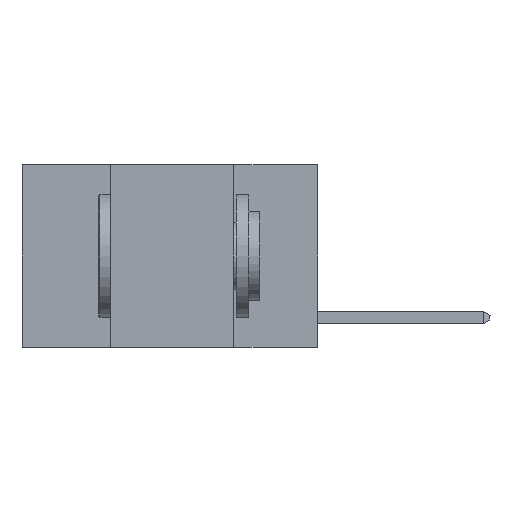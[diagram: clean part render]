
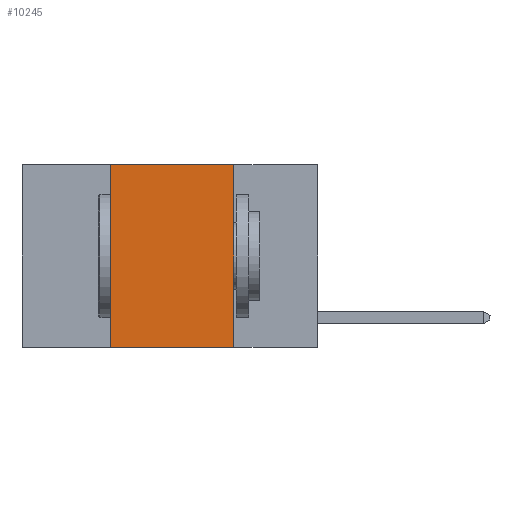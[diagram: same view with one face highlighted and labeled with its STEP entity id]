
A CAD part, left-side view. The second image highlights one B-rep face of the part: STEP entity #10245.
In plain terms, the highlighted planar face has unit normal (-1, 0, 0).
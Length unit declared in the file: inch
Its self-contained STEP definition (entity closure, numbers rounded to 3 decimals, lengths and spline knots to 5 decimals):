
#399 = CARTESIAN_POINT ( 'NONE',  ( 0., 0.42, 0. ) ) ;
#499 = VECTOR ( 'NONE', #5237, 39.37008 ) ;
#953 = ORIENTED_EDGE ( 'NONE', *, *, #14781, .F. ) ;
#2214 = EDGE_CURVE ( 'NONE', #9195, #16380, #9853, .T. ) ;
#2644 = EDGE_CURVE ( 'NONE', #16380, #14195, #6118, .T. ) ;
#5237 = DIRECTION ( 'NONE',  ( 0., 0., 1. ) ) ;
#5583 = VECTOR ( 'NONE', #18920, 39.37008 ) ;
#5860 = DIRECTION ( 'NONE',  ( 0., 0., -1. ) ) ;
#6118 = LINE ( 'NONE', #16441, #20016 ) ;
#6196 = DIRECTION ( 'NONE',  ( 0., -1., 0. ) ) ;
#6877 = CARTESIAN_POINT ( 'NONE',  ( 0., 0.42, -0.37 ) ) ;
#8248 = VERTEX_POINT ( 'NONE', #22944 ) ;
#8418 = LINE ( 'NONE', #15172, #11577 ) ;
#9195 = VERTEX_POINT ( 'NONE', #6877 ) ;
#9631 = ORIENTED_EDGE ( 'NONE', *, *, #11761, .T. ) ;
#9853 = LINE ( 'NONE', #22714, #499 ) ;
#10245 = ADVANCED_FACE ( 'NONE', ( #18081 ), #11135, .F. ) ;
#11135 = PLANE ( 'NONE',  #13983 ) ;
#11577 = VECTOR ( 'NONE', #6196, 39.37008 ) ;
#11761 = EDGE_CURVE ( 'NONE', #9195, #8248, #8418, .T. ) ;
#13805 = ORIENTED_EDGE ( 'NONE', *, *, #2644, .F. ) ;
#13983 = AXIS2_PLACEMENT_3D ( 'NONE', #16657, #20519, #5860 ) ;
#14137 = EDGE_LOOP ( 'NONE', ( #953, #13805, #22212, #9631 ) ) ;
#14195 = VERTEX_POINT ( 'NONE', #18393 ) ;
#14781 = EDGE_CURVE ( 'NONE', #14195, #8248, #20051, .T. ) ;
#15172 = CARTESIAN_POINT ( 'NONE',  ( 0., 0.6, -0.37 ) ) ;
#16380 = VERTEX_POINT ( 'NONE', #399 ) ;
#16441 = CARTESIAN_POINT ( 'NONE',  ( 0., 0.6, 0. ) ) ;
#16657 = CARTESIAN_POINT ( 'NONE',  ( 0., 0.6, 0. ) ) ;
#17093 = CARTESIAN_POINT ( 'NONE',  ( 0., 0.17, 0. ) ) ;
#18081 = FACE_OUTER_BOUND ( 'NONE', #14137, .T. ) ;
#18331 = DIRECTION ( 'NONE',  ( 0., -1., 0. ) ) ;
#18393 = CARTESIAN_POINT ( 'NONE',  ( 0., 0.17, 0. ) ) ;
#18920 = DIRECTION ( 'NONE',  ( 0., 0., -1. ) ) ;
#20016 = VECTOR ( 'NONE', #18331, 39.37008 ) ;
#20051 = LINE ( 'NONE', #17093, #5583 ) ;
#20519 = DIRECTION ( 'NONE',  ( 1., 0., 0. ) ) ;
#22212 = ORIENTED_EDGE ( 'NONE', *, *, #2214, .F. ) ;
#22714 = CARTESIAN_POINT ( 'NONE',  ( 0., 0.42, 0. ) ) ;
#22944 = CARTESIAN_POINT ( 'NONE',  ( 0., 0.17, -0.37 ) ) ;
